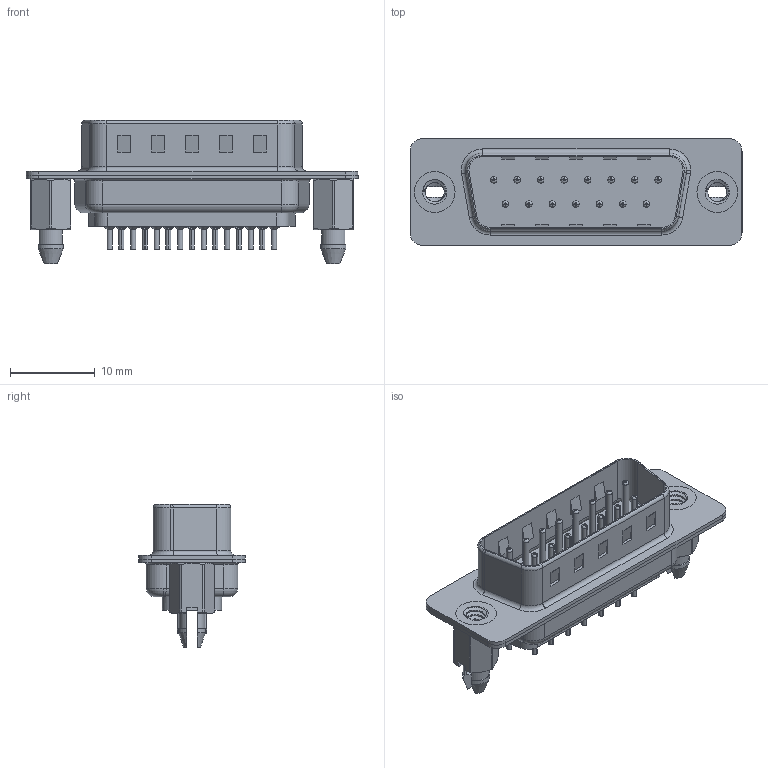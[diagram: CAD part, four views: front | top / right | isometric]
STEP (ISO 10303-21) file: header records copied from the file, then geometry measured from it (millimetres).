
FILE_DESCRIPTION (( 'STEP AP203' ), '1' );
FILE_NAME ('627-015-220-546.STEP', '2018-10-04T01:01:46', ( '' ), ( '' ), 'SwSTEP 2.0', 'SolidWorks 2016', '' );
FILE_SCHEMA (( 'CONFIG_CONTROL_DESIGN' ));
Length unit declared in the file: millimetre
Products named in the file (7): 627-015-220-546; 627 Housing_15 LP; 627 Shell Front_15 Contacts; 627 Shell Rear_15 Contacts; 627 Contact Row 1_20L; 627 Contact Row 2_20L; 627 4-40 Threaded Boardlock_LP
Assembly tree (20 placements, depth 2):
  627-015-220-546
    627 Housing_15 LP
    627 Shell Front_15 Contacts
    627 Shell Rear_15 Contacts
    627 Contact Row 1_20L  x8
    627 Contact Row 2_20L  x7
    627 4-40 Threaded Boardlock_LP  x2
Bounding box: 39.15 x 12.6 x 16.9 mm (x, y, z)
Volume: 1937.7 mm3; surface area: 5592.9 mm2
Topology: 20 solids, 20 shells, 1884 faces, 4946 edges, 3081 vertices
Faces by surface type: cylinder 720, plane 531, torus 461, cone 166, bspline 6
Entity records: 22468 total; most frequent: CARTESIAN_POINT 5363, DIRECTION 3536, ORIENTED_EDGE 3266, EDGE_CURVE 1633, AXIS2_PLACEMENT_3D 1394, VERTEX_POINT 1039, VECTOR 748, LINE 748
